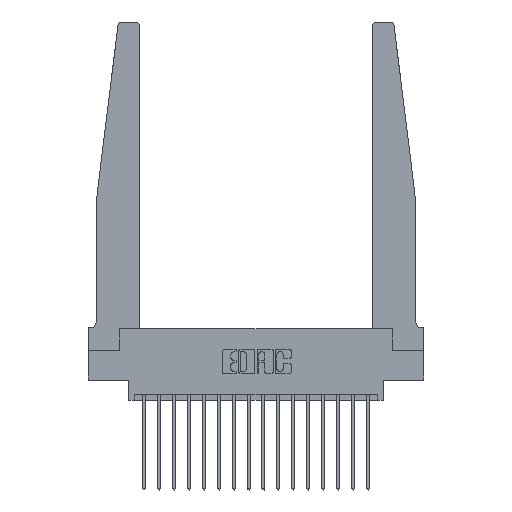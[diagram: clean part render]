
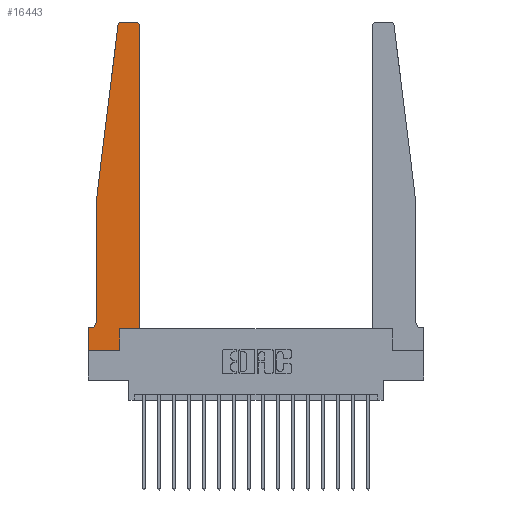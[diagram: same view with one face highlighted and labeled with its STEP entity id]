
A CAD part, top view. The second image highlights one B-rep face of the part: STEP entity #16443.
In plain terms, the highlighted planar face has unit normal (0, 0, 1).
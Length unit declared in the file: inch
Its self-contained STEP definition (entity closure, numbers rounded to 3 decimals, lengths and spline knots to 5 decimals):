
#41 = DIRECTION ( 'NONE',  ( 0., -1., 0. ) ) ;
#63 = DIRECTION ( 'NONE',  ( 1., 0., 0. ) ) ;
#353 = ORIENTED_EDGE ( 'NONE', *, *, #18606, .T. ) ;
#444 = CARTESIAN_POINT ( 'NONE',  ( 0.395, 2.75, 0.37 ) ) ;
#477 = CARTESIAN_POINT ( 'NONE',  ( 0.065, 1.25, 0.37 ) ) ;
#601 = CARTESIAN_POINT ( 'NONE',  ( 0.2605, 0.18, 0.37 ) ) ;
#624 = DIRECTION ( 'NONE',  ( -1., 0., 0. ) ) ;
#1185 = LINE ( 'NONE', #6858, #12388 ) ;
#1319 = EDGE_CURVE ( 'NONE', #6672, #11901, #13872, .T. ) ;
#1487 = CARTESIAN_POINT ( 'NONE',  ( 0.27653, 2.75, 0.37 ) ) ;
#1722 = CARTESIAN_POINT ( 'NONE',  ( 0.425, 0.18, 0.37 ) ) ;
#2129 = CARTESIAN_POINT ( 'NONE',  ( 0.425, 2.72, 0.37 ) ) ;
#2521 = VERTEX_POINT ( 'NONE', #10815 ) ;
#2664 = VECTOR ( 'NONE', #4973, 39.37008 ) ;
#2746 = ORIENTED_EDGE ( 'NONE', *, *, #14972, .T. ) ;
#2862 = ORIENTED_EDGE ( 'NONE', *, *, #6158, .T. ) ;
#3021 = LINE ( 'NONE', #13727, #10753 ) ;
#3037 = CARTESIAN_POINT ( 'NONE',  ( 0., 0.1875, 0.37 ) ) ;
#3279 = AXIS2_PLACEMENT_3D ( 'NONE', #18082, #9307, #624 ) ;
#3281 = AXIS2_PLACEMENT_3D ( 'NONE', #5838, #8763, #63 ) ;
#3614 = CARTESIAN_POINT ( 'NONE',  ( 0.25, 2.75, 0.37 ) ) ;
#3773 = EDGE_CURVE ( 'NONE', #14658, #6672, #17457, .T. ) ;
#3921 = VECTOR ( 'NONE', #15295, 39.37008 ) ;
#3991 = ORIENTED_EDGE ( 'NONE', *, *, #15665, .T. ) ;
#4037 = ORIENTED_EDGE ( 'NONE', *, *, #3773, .T. ) ;
#4369 = PLANE ( 'NONE',  #3281 ) ;
#4378 = LINE ( 'NONE', #9359, #3921 ) ;
#4421 = FACE_OUTER_BOUND ( 'NONE', #18018, .T. ) ;
#4973 = DIRECTION ( 'NONE',  ( 1., 0., 0. ) ) ;
#5076 = EDGE_CURVE ( 'NONE', #11640, #15155, #1185, .T. ) ;
#5292 = VECTOR ( 'NONE', #6373, 39.37008 ) ;
#5457 = DIRECTION ( 'NONE',  ( 1., 0., 0. ) ) ;
#5510 = EDGE_CURVE ( 'NONE', #2521, #8930, #13745, .T. ) ;
#5838 = CARTESIAN_POINT ( 'NONE',  ( 0., 0.1875, 0.37 ) ) ;
#5869 = EDGE_CURVE ( 'NONE', #11901, #2521, #18499, .T. ) ;
#6029 = ORIENTED_EDGE ( 'NONE', *, *, #5869, .T. ) ;
#6051 = AXIS2_PLACEMENT_3D ( 'NONE', #6657, #16904, #8132 ) ;
#6063 = VECTOR ( 'NONE', #12851, 39.37008 ) ;
#6158 = EDGE_CURVE ( 'NONE', #14503, #11640, #14869, .T. ) ;
#6373 = DIRECTION ( 'NONE',  ( -1., 0., 0. ) ) ;
#6657 = CARTESIAN_POINT ( 'NONE',  ( 0.27653, 2.72, 0.37 ) ) ;
#6671 = LINE ( 'NONE', #3614, #14032 ) ;
#6672 = VERTEX_POINT ( 'NONE', #17673 ) ;
#6747 = CARTESIAN_POINT ( 'NONE',  ( 0.395, 2.72, 0.37 ) ) ;
#6755 = VERTEX_POINT ( 'NONE', #444 ) ;
#6858 = CARTESIAN_POINT ( 'NONE',  ( 0.425, 0.18, 0.37 ) ) ;
#7842 = DIRECTION ( 'NONE',  ( 0., 1., 0. ) ) ;
#8132 = DIRECTION ( 'NONE',  ( 1., 0., 0. ) ) ;
#8218 = DIRECTION ( 'NONE',  ( 1., 0., 0. ) ) ;
#8370 = EDGE_CURVE ( 'NONE', #9341, #14180, #3021, .T. ) ;
#8763 = DIRECTION ( 'NONE',  ( 0., 0., 1. ) ) ;
#8930 = VERTEX_POINT ( 'NONE', #13905 ) ;
#9240 = CARTESIAN_POINT ( 'NONE',  ( 0.065, 0.1875, 0.37 ) ) ;
#9254 = CIRCLE ( 'NONE', #9980, 0.03 ) ;
#9307 = DIRECTION ( 'NONE',  ( 0., 0., -1. ) ) ;
#9341 = VERTEX_POINT ( 'NONE', #3037 ) ;
#9348 = CARTESIAN_POINT ( 'NONE',  ( 0., 0., 0.37 ) ) ;
#9359 = CARTESIAN_POINT ( 'NONE',  ( 0.425, 0.18, 0.37 ) ) ;
#9465 = DIRECTION ( 'NONE',  ( -1., 0., 0. ) ) ;
#9621 = LINE ( 'NONE', #9240, #5292 ) ;
#9738 = ORIENTED_EDGE ( 'NONE', *, *, #18013, .T. ) ;
#9935 = LINE ( 'NONE', #9348, #2664 ) ;
#9980 = AXIS2_PLACEMENT_3D ( 'NONE', #6747, #16990, #8218 ) ;
#10171 = VERTEX_POINT ( 'NONE', #2129 ) ;
#10678 = CARTESIAN_POINT ( 'NONE',  ( 0., 0., 0.37 ) ) ;
#10728 = VECTOR ( 'NONE', #41, 39.37008 ) ;
#10753 = VECTOR ( 'NONE', #12316, 39.37008 ) ;
#10815 = CARTESIAN_POINT ( 'NONE',  ( 0.065, 0.2375, 0.37 ) ) ;
#11532 = ORIENTED_EDGE ( 'NONE', *, *, #8370, .T. ) ;
#11640 = VERTEX_POINT ( 'NONE', #17401 ) ;
#11901 = VERTEX_POINT ( 'NONE', #477 ) ;
#12291 = ORIENTED_EDGE ( 'NONE', *, *, #1319, .T. ) ;
#12316 = DIRECTION ( 'NONE',  ( 0., -1., 0. ) ) ;
#12388 = VECTOR ( 'NONE', #5457, 39.37008 ) ;
#12851 = DIRECTION ( 'NONE',  ( -0.122, -0.992, 0. ) ) ;
#13124 = CARTESIAN_POINT ( 'NONE',  ( 0.065, 1.25, 0.37 ) ) ;
#13638 = CARTESIAN_POINT ( 'NONE',  ( 0.065, 1.25, 0.37 ) ) ;
#13727 = CARTESIAN_POINT ( 'NONE',  ( 0., 0., 0.37 ) ) ;
#13745 = CIRCLE ( 'NONE', #3279, 0.05 ) ;
#13872 = LINE ( 'NONE', #13638, #6063 ) ;
#13905 = CARTESIAN_POINT ( 'NONE',  ( 0.015, 0.1875, 0.37 ) ) ;
#14032 = VECTOR ( 'NONE', #9465, 39.37008 ) ;
#14180 = VERTEX_POINT ( 'NONE', #10678 ) ;
#14429 = VECTOR ( 'NONE', #7842, 39.37008 ) ;
#14503 = VERTEX_POINT ( 'NONE', #15764 ) ;
#14658 = VERTEX_POINT ( 'NONE', #1487 ) ;
#14869 = LINE ( 'NONE', #601, #14429 ) ;
#14972 = EDGE_CURVE ( 'NONE', #10171, #6755, #9254, .T. ) ;
#15155 = VERTEX_POINT ( 'NONE', #1722 ) ;
#15295 = DIRECTION ( 'NONE',  ( 0., 1., 0. ) ) ;
#15665 = EDGE_CURVE ( 'NONE', #14180, #14503, #9935, .T. ) ;
#15764 = CARTESIAN_POINT ( 'NONE',  ( 0.2605, 0., 0.37 ) ) ;
#16443 = ADVANCED_FACE ( 'NONE', ( #4421 ), #4369, .T. ) ;
#16904 = DIRECTION ( 'NONE',  ( 0., 0., 1. ) ) ;
#16990 = DIRECTION ( 'NONE',  ( 0., 0., 1. ) ) ;
#17121 = ORIENTED_EDGE ( 'NONE', *, *, #18680, .T. ) ;
#17289 = ORIENTED_EDGE ( 'NONE', *, *, #5510, .T. ) ;
#17401 = CARTESIAN_POINT ( 'NONE',  ( 0.2605, 0.18, 0.37 ) ) ;
#17457 = CIRCLE ( 'NONE', #6051, 0.03 ) ;
#17673 = CARTESIAN_POINT ( 'NONE',  ( 0.24675, 2.72367, 0.37 ) ) ;
#17915 = ORIENTED_EDGE ( 'NONE', *, *, #5076, .T. ) ;
#18013 = EDGE_CURVE ( 'NONE', #6755, #14658, #6671, .T. ) ;
#18018 = EDGE_LOOP ( 'NONE', ( #9738, #4037, #12291, #6029, #17289, #353, #11532, #3991, #2862, #17915, #17121, #2746 ) ) ;
#18082 = CARTESIAN_POINT ( 'NONE',  ( 0.015, 0.2375, 0.37 ) ) ;
#18499 = LINE ( 'NONE', #13124, #10728 ) ;
#18606 = EDGE_CURVE ( 'NONE', #8930, #9341, #9621, .T. ) ;
#18680 = EDGE_CURVE ( 'NONE', #15155, #10171, #4378, .T. ) ;
